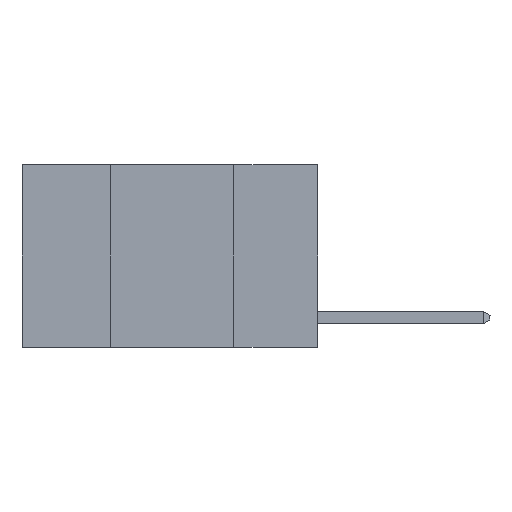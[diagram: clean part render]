
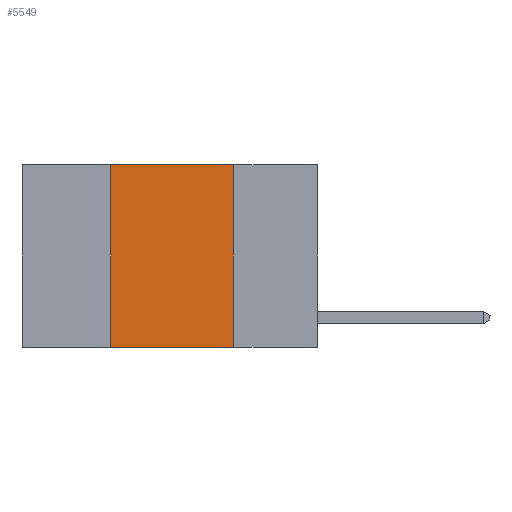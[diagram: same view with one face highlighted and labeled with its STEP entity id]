
A CAD part, left-side view. The second image highlights one B-rep face of the part: STEP entity #5549.
In plain terms, the highlighted planar face has unit normal (-1, 0, 0).
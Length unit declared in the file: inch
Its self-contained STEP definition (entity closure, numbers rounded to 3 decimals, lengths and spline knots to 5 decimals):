
#142 = VECTOR ( 'NONE', #5015, 39.37008 ) ;
#332 = CARTESIAN_POINT ( 'NONE',  ( 0., 0.42, 0. ) ) ;
#696 = EDGE_CURVE ( 'NONE', #1776, #3215, #9049, .T. ) ;
#740 = CARTESIAN_POINT ( 'NONE',  ( 0., 0.42, 0. ) ) ;
#1776 = VERTEX_POINT ( 'NONE', #7660 ) ;
#1832 = DIRECTION ( 'NONE',  ( 1., 0., 0. ) ) ;
#3172 = ORIENTED_EDGE ( 'NONE', *, *, #13484, .F. ) ;
#3215 = VERTEX_POINT ( 'NONE', #14846 ) ;
#3746 = AXIS2_PLACEMENT_3D ( 'NONE', #10321, #1832, #5399 ) ;
#4080 = CARTESIAN_POINT ( 'NONE',  ( 0., 0.42, -0.37 ) ) ;
#4363 = DIRECTION ( 'NONE',  ( 0., 0., -1. ) ) ;
#4727 = EDGE_LOOP ( 'NONE', ( #9039, #3172, #11961, #5136 ) ) ;
#5015 = DIRECTION ( 'NONE',  ( 0., -1., 0. ) ) ;
#5107 = EDGE_CURVE ( 'NONE', #14192, #5817, #7589, .T. ) ;
#5136 = ORIENTED_EDGE ( 'NONE', *, *, #6550, .T. ) ;
#5399 = DIRECTION ( 'NONE',  ( 0., 0., -1. ) ) ;
#5513 = CARTESIAN_POINT ( 'NONE',  ( 0., 0.6, -0.37 ) ) ;
#5549 = ADVANCED_FACE ( 'NONE', ( #11555 ), #10204, .F. ) ;
#5817 = VERTEX_POINT ( 'NONE', #332 ) ;
#6528 = DIRECTION ( 'NONE',  ( 0., -1., 0. ) ) ;
#6550 = EDGE_CURVE ( 'NONE', #14192, #3215, #14530, .T. ) ;
#7589 = LINE ( 'NONE', #740, #12702 ) ;
#7660 = CARTESIAN_POINT ( 'NONE',  ( 0., 0.17, 0. ) ) ;
#9039 = ORIENTED_EDGE ( 'NONE', *, *, #696, .F. ) ;
#9049 = LINE ( 'NONE', #14131, #13213 ) ;
#10204 = PLANE ( 'NONE',  #3746 ) ;
#10321 = CARTESIAN_POINT ( 'NONE',  ( 0., 0.6, 0. ) ) ;
#10563 = VECTOR ( 'NONE', #6528, 39.37008 ) ;
#11555 = FACE_OUTER_BOUND ( 'NONE', #4727, .T. ) ;
#11961 = ORIENTED_EDGE ( 'NONE', *, *, #5107, .F. ) ;
#12647 = DIRECTION ( 'NONE',  ( 0., 0., 1. ) ) ;
#12702 = VECTOR ( 'NONE', #12647, 39.37008 ) ;
#12714 = LINE ( 'NONE', #13619, #142 ) ;
#13213 = VECTOR ( 'NONE', #4363, 39.37008 ) ;
#13484 = EDGE_CURVE ( 'NONE', #5817, #1776, #12714, .T. ) ;
#13619 = CARTESIAN_POINT ( 'NONE',  ( 0., 0.6, 0. ) ) ;
#14131 = CARTESIAN_POINT ( 'NONE',  ( 0., 0.17, 0. ) ) ;
#14192 = VERTEX_POINT ( 'NONE', #4080 ) ;
#14530 = LINE ( 'NONE', #5513, #10563 ) ;
#14846 = CARTESIAN_POINT ( 'NONE',  ( 0., 0.17, -0.37 ) ) ;
